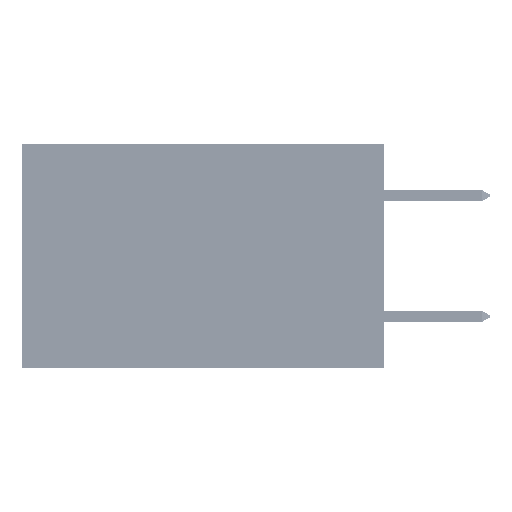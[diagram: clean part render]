
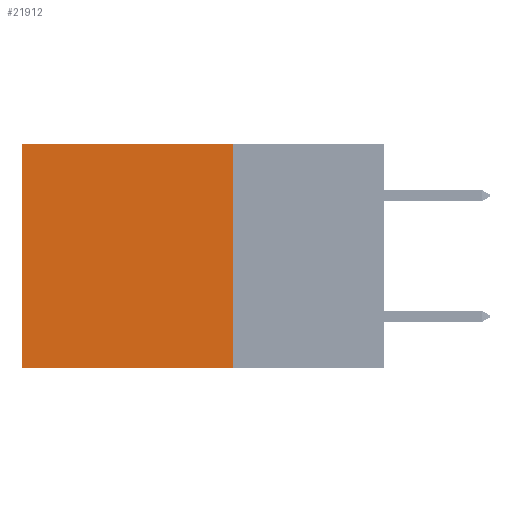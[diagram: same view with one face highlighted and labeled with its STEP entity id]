
A CAD part, left-side view. The second image highlights one B-rep face of the part: STEP entity #21912.
In plain terms, the highlighted planar face has unit normal (-1, 0, 0).
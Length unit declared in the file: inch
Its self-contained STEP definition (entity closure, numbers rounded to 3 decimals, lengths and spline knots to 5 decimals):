
#646 = EDGE_CURVE ( 'NONE', #14061, #35468, #28116, .T. ) ;
#1111 = ORIENTED_EDGE ( 'NONE', *, *, #646, .F. ) ;
#1115 = EDGE_CURVE ( 'NONE', #48375, #35468, #5674, .T. ) ;
#3195 = CARTESIAN_POINT ( 'NONE',  ( 0.2875, 0.6, -0.37 ) ) ;
#4472 = DIRECTION ( 'NONE',  ( 0., 0., -1. ) ) ;
#5674 = LINE ( 'NONE', #30988, #8713 ) ;
#5905 = DIRECTION ( 'NONE',  ( 0., 1., 0. ) ) ;
#7121 = LINE ( 'NONE', #26126, #27704 ) ;
#7445 = CARTESIAN_POINT ( 'NONE',  ( 0.2875, 0.6, 0. ) ) ;
#7540 = VECTOR ( 'NONE', #47997, 39.37008 ) ;
#8337 = PLANE ( 'NONE',  #31161 ) ;
#8713 = VECTOR ( 'NONE', #11702, 39.37008 ) ;
#8785 = EDGE_LOOP ( 'NONE', ( #31690, #1111, #16993, #43168 ) ) ;
#10669 = CARTESIAN_POINT ( 'NONE',  ( 0.2875, 0.25, -0.37 ) ) ;
#11702 = DIRECTION ( 'NONE',  ( 0., 0., -1. ) ) ;
#14061 = VERTEX_POINT ( 'NONE', #10669 ) ;
#16354 = EDGE_CURVE ( 'NONE', #43587, #14061, #7121, .T. ) ;
#16993 = ORIENTED_EDGE ( 'NONE', *, *, #16354, .F. ) ;
#21912 = ADVANCED_FACE ( 'NONE', ( #25226 ), #8337, .F. ) ;
#22521 = EDGE_CURVE ( 'NONE', #43587, #48375, #40269, .T. ) ;
#24040 = DIRECTION ( 'NONE',  ( 0., 0., -1. ) ) ;
#25226 = FACE_OUTER_BOUND ( 'NONE', #8785, .T. ) ;
#26126 = CARTESIAN_POINT ( 'NONE',  ( 0.2875, 0.25, 0. ) ) ;
#27704 = VECTOR ( 'NONE', #4472, 39.37008 ) ;
#27957 = DIRECTION ( 'NONE',  ( 1., 0., 0. ) ) ;
#28116 = LINE ( 'NONE', #28756, #7540 ) ;
#28213 = CARTESIAN_POINT ( 'NONE',  ( 0.2875, 0.25, 0. ) ) ;
#28756 = CARTESIAN_POINT ( 'NONE',  ( 0.2875, 0.25, -0.37 ) ) ;
#30615 = VECTOR ( 'NONE', #5905, 39.37008 ) ;
#30988 = CARTESIAN_POINT ( 'NONE',  ( 0.2875, 0.6, 0. ) ) ;
#31161 = AXIS2_PLACEMENT_3D ( 'NONE', #47185, #27957, #24040 ) ;
#31690 = ORIENTED_EDGE ( 'NONE', *, *, #1115, .T. ) ;
#35468 = VERTEX_POINT ( 'NONE', #3195 ) ;
#40269 = LINE ( 'NONE', #46290, #30615 ) ;
#43168 = ORIENTED_EDGE ( 'NONE', *, *, #22521, .T. ) ;
#43587 = VERTEX_POINT ( 'NONE', #28213 ) ;
#46290 = CARTESIAN_POINT ( 'NONE',  ( 0.2875, 0.25, 0. ) ) ;
#47185 = CARTESIAN_POINT ( 'NONE',  ( 0.2875, 0.25, 0. ) ) ;
#47997 = DIRECTION ( 'NONE',  ( 0., 1., 0. ) ) ;
#48375 = VERTEX_POINT ( 'NONE', #7445 ) ;
